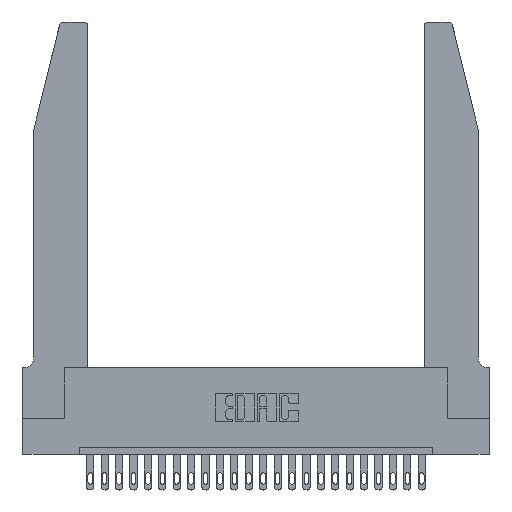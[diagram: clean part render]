
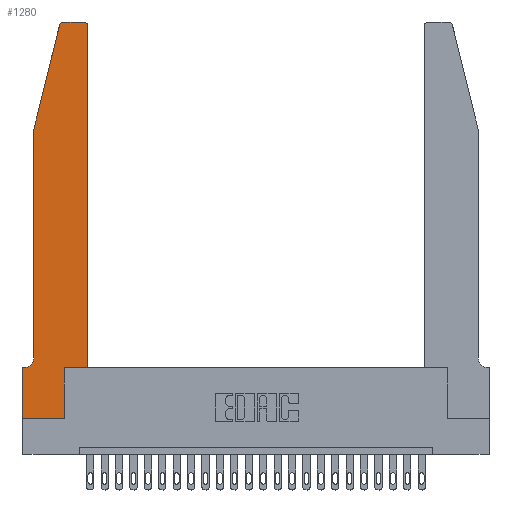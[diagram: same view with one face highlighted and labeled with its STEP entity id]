
A CAD part, top view. The second image highlights one B-rep face of the part: STEP entity #1280.
In plain terms, the highlighted planar face has unit normal (0, 0, 1).
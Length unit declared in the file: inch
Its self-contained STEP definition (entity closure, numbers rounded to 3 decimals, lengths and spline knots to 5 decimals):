
#48 = VERTEX_POINT ( 'NONE', #9289 ) ;
#91 = DIRECTION ( 'NONE',  ( -1., 0., 0. ) ) ;
#133 = EDGE_CURVE ( 'NONE', #8063, #21507, #396, .T. ) ;
#252 = ORIENTED_EDGE ( 'NONE', *, *, #21182, .T. ) ;
#396 = CIRCLE ( 'NONE', #23736, 0.03 ) ;
#480 = ORIENTED_EDGE ( 'NONE', *, *, #23943, .T. ) ;
#657 = VERTEX_POINT ( 'NONE', #10722 ) ;
#703 = CARTESIAN_POINT ( 'NONE',  ( 0.284, 2.72, 0.37 ) ) ;
#892 = VECTOR ( 'NONE', #12086, 39.37008 ) ;
#1079 = DIRECTION ( 'NONE',  ( -1., 0., 0. ) ) ;
#1199 = LINE ( 'NONE', #12259, #892 ) ;
#1270 = VERTEX_POINT ( 'NONE', #18885 ) ;
#1280 = ADVANCED_FACE ( 'NONE', ( #12845 ), #22785, .T. ) ;
#2083 = VECTOR ( 'NONE', #24703, 39.37008 ) ;
#2959 = EDGE_LOOP ( 'NONE', ( #22058, #23049, #19525, #15581, #16015, #14527, #12926, #252, #480, #13681, #24424, #17426 ) ) ;
#3312 = AXIS2_PLACEMENT_3D ( 'NONE', #703, #12523, #8645 ) ;
#3971 = LINE ( 'NONE', #14658, #7049 ) ;
#4322 = LINE ( 'NONE', #24403, #24411 ) ;
#4577 = EDGE_CURVE ( 'NONE', #16557, #25075, #16297, .T. ) ;
#4716 = CARTESIAN_POINT ( 'NONE',  ( 0.2865, 0.35, 0.37 ) ) ;
#5037 = CIRCLE ( 'NONE', #3312, 0.03 ) ;
#5121 = CARTESIAN_POINT ( 'NONE',  ( 0.4505, 0.35, 0.37 ) ) ;
#5962 = CARTESIAN_POINT ( 'NONE',  ( 0.4205, 2.72, 0.37 ) ) ;
#6017 = CARTESIAN_POINT ( 'NONE',  ( 0.2865, 0.35, 0.37 ) ) ;
#6105 = LINE ( 'NONE', #7597, #17936 ) ;
#6420 = EDGE_CURVE ( 'NONE', #657, #16557, #24255, .T. ) ;
#6577 = VECTOR ( 'NONE', #24181, 39.37008 ) ;
#7049 = VECTOR ( 'NONE', #9276, 39.37008 ) ;
#7059 = VERTEX_POINT ( 'NONE', #16530 ) ;
#7105 = LINE ( 'NONE', #9653, #25022 ) ;
#7597 = CARTESIAN_POINT ( 'NONE',  ( 0.0755, 2., 0.37 ) ) ;
#8063 = VERTEX_POINT ( 'NONE', #24572 ) ;
#8074 = VERTEX_POINT ( 'NONE', #5121 ) ;
#8147 = DIRECTION ( 'NONE',  ( 1., 0., 0. ) ) ;
#8645 = DIRECTION ( 'NONE',  ( 1., 0., 0. ) ) ;
#9110 = LINE ( 'NONE', #11096, #2083 ) ;
#9193 = LINE ( 'NONE', #10785, #14921 ) ;
#9276 = DIRECTION ( 'NONE',  ( 1., 0., 0. ) ) ;
#9289 = CARTESIAN_POINT ( 'NONE',  ( 0., 0., 0.37 ) ) ;
#9653 = CARTESIAN_POINT ( 'NONE',  ( 0.2605, 2.75, 0.37 ) ) ;
#9702 = DIRECTION ( 'NONE',  ( -0.239, -0.971, 0. ) ) ;
#9900 = CARTESIAN_POINT ( 'NONE',  ( 0.0055, 0.42, 0.37 ) ) ;
#10571 = VECTOR ( 'NONE', #22063, 39.37008 ) ;
#10722 = CARTESIAN_POINT ( 'NONE',  ( 0.0755, 2., 0.37 ) ) ;
#10785 = CARTESIAN_POINT ( 'NONE',  ( 0.0755, 0.35, 0.37 ) ) ;
#10839 = VERTEX_POINT ( 'NONE', #25059 ) ;
#10946 = EDGE_CURVE ( 'NONE', #25075, #7059, #9193, .T. ) ;
#11096 = CARTESIAN_POINT ( 'NONE',  ( 0., 0., 0.37 ) ) ;
#11351 = EDGE_CURVE ( 'NONE', #10839, #657, #6105, .T. ) ;
#12086 = DIRECTION ( 'NONE',  ( 0., 1., 0. ) ) ;
#12259 = CARTESIAN_POINT ( 'NONE',  ( 0.4505, 0.35, 0.37 ) ) ;
#12523 = DIRECTION ( 'NONE',  ( 0., 0., 1. ) ) ;
#12700 = EDGE_CURVE ( 'NONE', #12944, #10839, #5037, .T. ) ;
#12845 = FACE_OUTER_BOUND ( 'NONE', #2959, .T. ) ;
#12876 = DIRECTION ( 'NONE',  ( 0., 0., 1. ) ) ;
#12926 = ORIENTED_EDGE ( 'NONE', *, *, #22150, .T. ) ;
#12944 = VERTEX_POINT ( 'NONE', #24499 ) ;
#13681 = ORIENTED_EDGE ( 'NONE', *, *, #19575, .T. ) ;
#14527 = ORIENTED_EDGE ( 'NONE', *, *, #10946, .T. ) ;
#14658 = CARTESIAN_POINT ( 'NONE',  ( 0., 0., 0.37 ) ) ;
#14735 = LINE ( 'NONE', #4716, #6577 ) ;
#14921 = VECTOR ( 'NONE', #1079, 39.37008 ) ;
#15581 = ORIENTED_EDGE ( 'NONE', *, *, #6420, .T. ) ;
#15725 = VERTEX_POINT ( 'NONE', #6017 ) ;
#15833 = DIRECTION ( 'NONE',  ( 0., 0., 1. ) ) ;
#16015 = ORIENTED_EDGE ( 'NONE', *, *, #4577, .T. ) ;
#16297 = CIRCLE ( 'NONE', #16927, 0.07 ) ;
#16530 = CARTESIAN_POINT ( 'NONE',  ( 0., 0.35, 0.37 ) ) ;
#16557 = VERTEX_POINT ( 'NONE', #23497 ) ;
#16927 = AXIS2_PLACEMENT_3D ( 'NONE', #9900, #23410, #91 ) ;
#17426 = ORIENTED_EDGE ( 'NONE', *, *, #133, .T. ) ;
#17936 = VECTOR ( 'NONE', #9702, 39.37008 ) ;
#18881 = AXIS2_PLACEMENT_3D ( 'NONE', #18958, #12876, #21005 ) ;
#18885 = CARTESIAN_POINT ( 'NONE',  ( 0.2865, 0., 0.37 ) ) ;
#18958 = CARTESIAN_POINT ( 'NONE',  ( 0., 0.35, 0.37 ) ) ;
#19055 = EDGE_CURVE ( 'NONE', #21507, #12944, #7105, .T. ) ;
#19525 = ORIENTED_EDGE ( 'NONE', *, *, #11351, .T. ) ;
#19575 = EDGE_CURVE ( 'NONE', #15725, #8074, #4322, .T. ) ;
#19818 = CARTESIAN_POINT ( 'NONE',  ( 0.4205, 2.75, 0.37 ) ) ;
#20896 = CARTESIAN_POINT ( 'NONE',  ( 0.0055, 0.35, 0.37 ) ) ;
#21005 = DIRECTION ( 'NONE',  ( 1., 0., 0. ) ) ;
#21182 = EDGE_CURVE ( 'NONE', #48, #1270, #3971, .T. ) ;
#21507 = VERTEX_POINT ( 'NONE', #19818 ) ;
#21528 = EDGE_CURVE ( 'NONE', #8074, #8063, #1199, .T. ) ;
#22058 = ORIENTED_EDGE ( 'NONE', *, *, #19055, .T. ) ;
#22063 = DIRECTION ( 'NONE',  ( 0., -1., 0. ) ) ;
#22150 = EDGE_CURVE ( 'NONE', #7059, #48, #9110, .T. ) ;
#22234 = CARTESIAN_POINT ( 'NONE',  ( 0.0755, 2., 0.37 ) ) ;
#22785 = PLANE ( 'NONE',  #18881 ) ;
#23049 = ORIENTED_EDGE ( 'NONE', *, *, #12700, .T. ) ;
#23260 = DIRECTION ( 'NONE',  ( -1., 0., 0. ) ) ;
#23308 = DIRECTION ( 'NONE',  ( 1., 0., 0. ) ) ;
#23410 = DIRECTION ( 'NONE',  ( 0., 0., -1. ) ) ;
#23497 = CARTESIAN_POINT ( 'NONE',  ( 0.0755, 0.42, 0.37 ) ) ;
#23736 = AXIS2_PLACEMENT_3D ( 'NONE', #5962, #15833, #8147 ) ;
#23943 = EDGE_CURVE ( 'NONE', #1270, #15725, #14735, .T. ) ;
#24181 = DIRECTION ( 'NONE',  ( 0., 1., 0. ) ) ;
#24255 = LINE ( 'NONE', #22234, #10571 ) ;
#24403 = CARTESIAN_POINT ( 'NONE',  ( 0.4505, 0.35, 0.37 ) ) ;
#24411 = VECTOR ( 'NONE', #23308, 39.37008 ) ;
#24424 = ORIENTED_EDGE ( 'NONE', *, *, #21528, .T. ) ;
#24499 = CARTESIAN_POINT ( 'NONE',  ( 0.284, 2.75, 0.37 ) ) ;
#24572 = CARTESIAN_POINT ( 'NONE',  ( 0.4505, 2.72, 0.37 ) ) ;
#24703 = DIRECTION ( 'NONE',  ( 0., -1., 0. ) ) ;
#25022 = VECTOR ( 'NONE', #23260, 39.37008 ) ;
#25059 = CARTESIAN_POINT ( 'NONE',  ( 0.25487, 2.72718, 0.37 ) ) ;
#25075 = VERTEX_POINT ( 'NONE', #20896 ) ;
